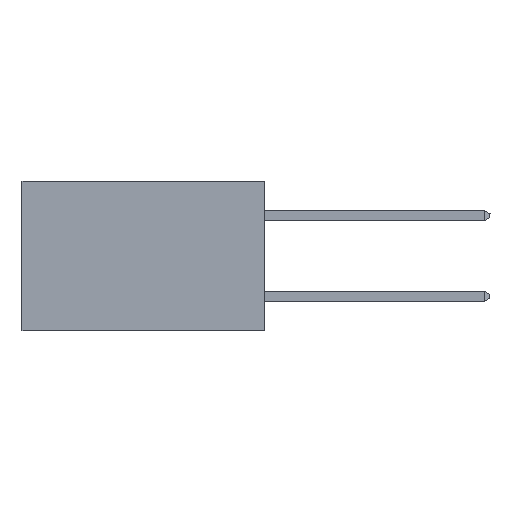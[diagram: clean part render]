
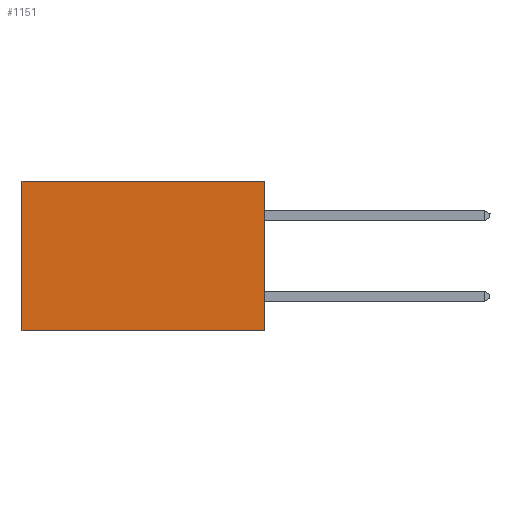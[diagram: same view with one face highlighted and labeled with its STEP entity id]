
A CAD part, left-side view. The second image highlights one B-rep face of the part: STEP entity #1151.
In plain terms, the highlighted planar face has unit normal (-1, 0, 0).
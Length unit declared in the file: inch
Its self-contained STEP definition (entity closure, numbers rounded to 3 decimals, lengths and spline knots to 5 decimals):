
#101 = CARTESIAN_POINT ( 'NONE',  ( 0.298, 0., -0.37 ) ) ;
#1151 = ADVANCED_FACE ( 'NONE', ( #5041 ), #28931, .F. ) ;
#1409 = ORIENTED_EDGE ( 'NONE', *, *, #1744, .F. ) ;
#1744 = EDGE_CURVE ( 'NONE', #24779, #30370, #24918, .T. ) ;
#1968 = LINE ( 'NONE', #11684, #9008 ) ;
#2777 = DIRECTION ( 'NONE',  ( 0., 0., -1. ) ) ;
#2964 = VECTOR ( 'NONE', #3293, 39.37008 ) ;
#3293 = DIRECTION ( 'NONE',  ( 0., 1., 0. ) ) ;
#3698 = LINE ( 'NONE', #29075, #2964 ) ;
#3947 = CARTESIAN_POINT ( 'NONE',  ( 0.298, 0., 0. ) ) ;
#5041 = FACE_OUTER_BOUND ( 'NONE', #21692, .T. ) ;
#6114 = VECTOR ( 'NONE', #2777, 39.37008 ) ;
#7857 = CARTESIAN_POINT ( 'NONE',  ( 0.298, 0.6, 0. ) ) ;
#8527 = CARTESIAN_POINT ( 'NONE',  ( 0.298, 0., 0. ) ) ;
#9008 = VECTOR ( 'NONE', #25732, 39.37008 ) ;
#11465 = VECTOR ( 'NONE', #16633, 39.37008 ) ;
#11684 = CARTESIAN_POINT ( 'NONE',  ( 0.298, 0.6, 0. ) ) ;
#11823 = CARTESIAN_POINT ( 'NONE',  ( 0.298, 0., -0.37 ) ) ;
#12016 = DIRECTION ( 'NONE',  ( 0., 0., -1. ) ) ;
#13768 = EDGE_CURVE ( 'NONE', #15965, #25532, #1968, .T. ) ;
#15965 = VERTEX_POINT ( 'NONE', #7857 ) ;
#16133 = ORIENTED_EDGE ( 'NONE', *, *, #16982, .T. ) ;
#16633 = DIRECTION ( 'NONE',  ( 0., 1., 0. ) ) ;
#16982 = EDGE_CURVE ( 'NONE', #24779, #15965, #3698, .T. ) ;
#17422 = EDGE_CURVE ( 'NONE', #30370, #25532, #27950, .T. ) ;
#18934 = CARTESIAN_POINT ( 'NONE',  ( 0.298, 0., 0. ) ) ;
#19792 = AXIS2_PLACEMENT_3D ( 'NONE', #8527, #30167, #12016 ) ;
#21692 = EDGE_LOOP ( 'NONE', ( #23361, #27304, #1409, #16133 ) ) ;
#23361 = ORIENTED_EDGE ( 'NONE', *, *, #13768, .T. ) ;
#24779 = VERTEX_POINT ( 'NONE', #3947 ) ;
#24918 = LINE ( 'NONE', #18934, #6114 ) ;
#25532 = VERTEX_POINT ( 'NONE', #25730 ) ;
#25730 = CARTESIAN_POINT ( 'NONE',  ( 0.298, 0.6, -0.37 ) ) ;
#25732 = DIRECTION ( 'NONE',  ( 0., 0., -1. ) ) ;
#27304 = ORIENTED_EDGE ( 'NONE', *, *, #17422, .F. ) ;
#27950 = LINE ( 'NONE', #101, #11465 ) ;
#28931 = PLANE ( 'NONE',  #19792 ) ;
#29075 = CARTESIAN_POINT ( 'NONE',  ( 0.298, 0., 0. ) ) ;
#30167 = DIRECTION ( 'NONE',  ( 1., 0., 0. ) ) ;
#30370 = VERTEX_POINT ( 'NONE', #11823 ) ;
